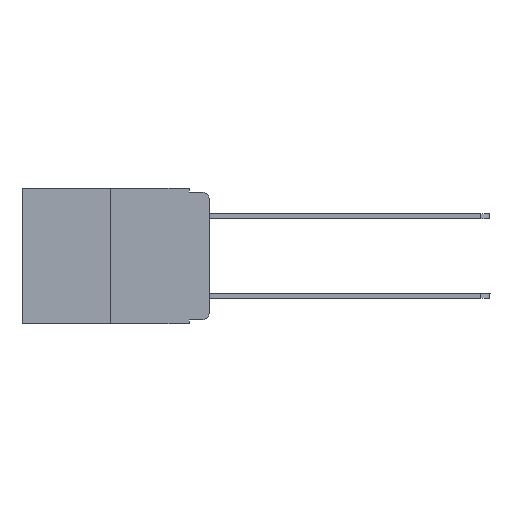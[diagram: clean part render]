
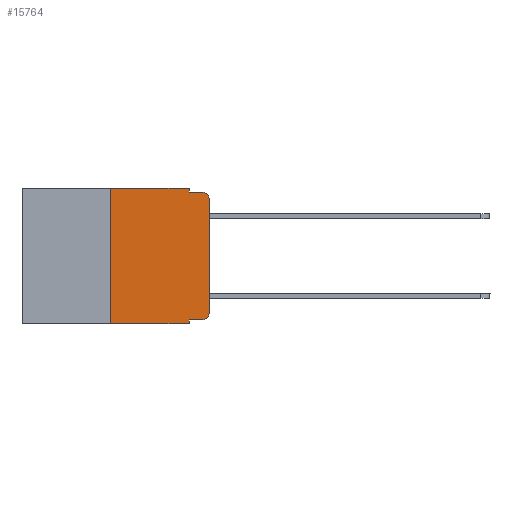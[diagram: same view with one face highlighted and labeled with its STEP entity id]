
A CAD part, left-side view. The second image highlights one B-rep face of the part: STEP entity #15764.
In plain terms, the highlighted planar face has unit normal (-1, 0, 0).
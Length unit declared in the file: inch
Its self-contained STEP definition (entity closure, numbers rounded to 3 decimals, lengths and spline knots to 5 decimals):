
#55 = LINE ( 'NONE', #3878, #13989 ) ;
#296 = LINE ( 'NONE', #6949, #2854 ) ;
#323 = LINE ( 'NONE', #3936, #1880 ) ;
#342 = CARTESIAN_POINT ( 'NONE',  ( 0., 0.473, 0. ) ) ;
#385 = AXIS2_PLACEMENT_3D ( 'NONE', #6421, #11253, #17907 ) ;
#438 = VECTOR ( 'NONE', #18726, 39.37008 ) ;
#1455 = DIRECTION ( 'NONE',  ( 0., -1., 0. ) ) ;
#1577 = VERTEX_POINT ( 'NONE', #8550 ) ;
#1880 = VECTOR ( 'NONE', #17052, 39.37008 ) ;
#2037 = EDGE_CURVE ( 'NONE', #3015, #19783, #8524, .T. ) ;
#2255 = CIRCLE ( 'NONE', #9578, 0.02 ) ;
#2854 = VECTOR ( 'NONE', #10037, 39.37008 ) ;
#3015 = VERTEX_POINT ( 'NONE', #21177 ) ;
#3674 = VERTEX_POINT ( 'NONE', #16917 ) ;
#3878 = CARTESIAN_POINT ( 'NONE',  ( 0., 0.25, 0. ) ) ;
#3936 = CARTESIAN_POINT ( 'NONE',  ( 0., 0.051, -0.333 ) ) ;
#4234 = DIRECTION ( 'NONE',  ( -1., 0., 0. ) ) ;
#4784 = FACE_OUTER_BOUND ( 'NONE', #13847, .T. ) ;
#4814 = CARTESIAN_POINT ( 'NONE',  ( 0., 0.02, -0.333 ) ) ;
#4974 = ORIENTED_EDGE ( 'NONE', *, *, #6089, .T. ) ;
#5379 = CARTESIAN_POINT ( 'NONE',  ( 0., 0.051, 0. ) ) ;
#5588 = VERTEX_POINT ( 'NONE', #20178 ) ;
#5590 = EDGE_CURVE ( 'NONE', #9705, #1577, #7108, .T. ) ;
#5601 = LINE ( 'NONE', #5379, #15461 ) ;
#5672 = EDGE_CURVE ( 'NONE', #5588, #14025, #5601, .T. ) ;
#5917 = VERTEX_POINT ( 'NONE', #4814 ) ;
#6089 = EDGE_CURVE ( 'NONE', #5588, #5917, #323, .T. ) ;
#6198 = VECTOR ( 'NONE', #8839, 39.37008 ) ;
#6421 = CARTESIAN_POINT ( 'NONE',  ( 0., 0.473, 0. ) ) ;
#6673 = EDGE_CURVE ( 'NONE', #19783, #3674, #2255, .T. ) ;
#6949 = CARTESIAN_POINT ( 'NONE',  ( 0., 0.473, -0.343 ) ) ;
#7108 = LINE ( 'NONE', #342, #438 ) ;
#8214 = CARTESIAN_POINT ( 'NONE',  ( 0., 0.25, 0. ) ) ;
#8524 = LINE ( 'NONE', #18594, #14614 ) ;
#8550 = CARTESIAN_POINT ( 'NONE',  ( 0., 0.051, 0. ) ) ;
#8839 = DIRECTION ( 'NONE',  ( 0., 0., -1. ) ) ;
#9578 = AXIS2_PLACEMENT_3D ( 'NONE', #19225, #4234, #19110 ) ;
#9705 = VERTEX_POINT ( 'NONE', #8214 ) ;
#9738 = CARTESIAN_POINT ( 'NONE',  ( 0., 0.051, -0.343 ) ) ;
#9891 = ORIENTED_EDGE ( 'NONE', *, *, #5590, .F. ) ;
#10037 = DIRECTION ( 'NONE',  ( 0., -1., 0. ) ) ;
#10203 = VERTEX_POINT ( 'NONE', #18697 ) ;
#10236 = EDGE_CURVE ( 'NONE', #1577, #10203, #20148, .T. ) ;
#10606 = DIRECTION ( 'NONE',  ( 0., 0., 1. ) ) ;
#10674 = ORIENTED_EDGE ( 'NONE', *, *, #16372, .F. ) ;
#11253 = DIRECTION ( 'NONE',  ( 1., 0., 0. ) ) ;
#11299 = ORIENTED_EDGE ( 'NONE', *, *, #6673, .T. ) ;
#12100 = VERTEX_POINT ( 'NONE', #17673 ) ;
#12112 = ORIENTED_EDGE ( 'NONE', *, *, #2037, .T. ) ;
#12249 = DIRECTION ( 'NONE',  ( 0., 0., -1. ) ) ;
#12337 = AXIS2_PLACEMENT_3D ( 'NONE', #18517, #18729, #15536 ) ;
#13532 = ORIENTED_EDGE ( 'NONE', *, *, #10236, .F. ) ;
#13750 = VECTOR ( 'NONE', #1455, 39.37008 ) ;
#13814 = ORIENTED_EDGE ( 'NONE', *, *, #5672, .F. ) ;
#13847 = EDGE_LOOP ( 'NONE', ( #12112, #11299, #16333, #13532, #9891, #10674, #20900, #13814, #4974, #18121 ) ) ;
#13869 = CARTESIAN_POINT ( 'NONE',  ( 0., 0.051, 0. ) ) ;
#13989 = VECTOR ( 'NONE', #15770, 39.37008 ) ;
#14025 = VERTEX_POINT ( 'NONE', #9738 ) ;
#14436 = CIRCLE ( 'NONE', #12337, 0.02 ) ;
#14614 = VECTOR ( 'NONE', #10606, 39.37008 ) ;
#15461 = VECTOR ( 'NONE', #12249, 39.37008 ) ;
#15536 = DIRECTION ( 'NONE',  ( 0., 0., -1. ) ) ;
#15764 = ADVANCED_FACE ( 'NONE', ( #4784 ), #21567, .F. ) ;
#15770 = DIRECTION ( 'NONE',  ( 0., 0., 1. ) ) ;
#15820 = EDGE_CURVE ( 'NONE', #12100, #14025, #296, .T. ) ;
#16333 = ORIENTED_EDGE ( 'NONE', *, *, #17822, .F. ) ;
#16372 = EDGE_CURVE ( 'NONE', #12100, #9705, #55, .T. ) ;
#16632 = CARTESIAN_POINT ( 'NONE',  ( 0., 0.051, -0.01 ) ) ;
#16917 = CARTESIAN_POINT ( 'NONE',  ( 0., 0.02, -0.01 ) ) ;
#17052 = DIRECTION ( 'NONE',  ( 0., -1., 0. ) ) ;
#17673 = CARTESIAN_POINT ( 'NONE',  ( 0., 0.25, -0.343 ) ) ;
#17822 = EDGE_CURVE ( 'NONE', #10203, #3674, #18407, .T. ) ;
#17902 = EDGE_CURVE ( 'NONE', #5917, #3015, #14436, .T. ) ;
#17907 = DIRECTION ( 'NONE',  ( 0., 0., -1. ) ) ;
#18121 = ORIENTED_EDGE ( 'NONE', *, *, #17902, .T. ) ;
#18407 = LINE ( 'NONE', #16632, #13750 ) ;
#18517 = CARTESIAN_POINT ( 'NONE',  ( 0., 0.02, -0.313 ) ) ;
#18594 = CARTESIAN_POINT ( 'NONE',  ( 0., 0., 0. ) ) ;
#18697 = CARTESIAN_POINT ( 'NONE',  ( 0., 0.051, -0.01 ) ) ;
#18726 = DIRECTION ( 'NONE',  ( 0., -1., 0. ) ) ;
#18729 = DIRECTION ( 'NONE',  ( -1., 0., 0. ) ) ;
#19110 = DIRECTION ( 'NONE',  ( 0., 0., -1. ) ) ;
#19225 = CARTESIAN_POINT ( 'NONE',  ( 0., 0.02, -0.03 ) ) ;
#19264 = CARTESIAN_POINT ( 'NONE',  ( 0., 0., -0.03 ) ) ;
#19783 = VERTEX_POINT ( 'NONE', #19264 ) ;
#20148 = LINE ( 'NONE', #13869, #6198 ) ;
#20178 = CARTESIAN_POINT ( 'NONE',  ( 0., 0.051, -0.333 ) ) ;
#20900 = ORIENTED_EDGE ( 'NONE', *, *, #15820, .T. ) ;
#21177 = CARTESIAN_POINT ( 'NONE',  ( 0., 0., -0.313 ) ) ;
#21567 = PLANE ( 'NONE',  #385 ) ;
